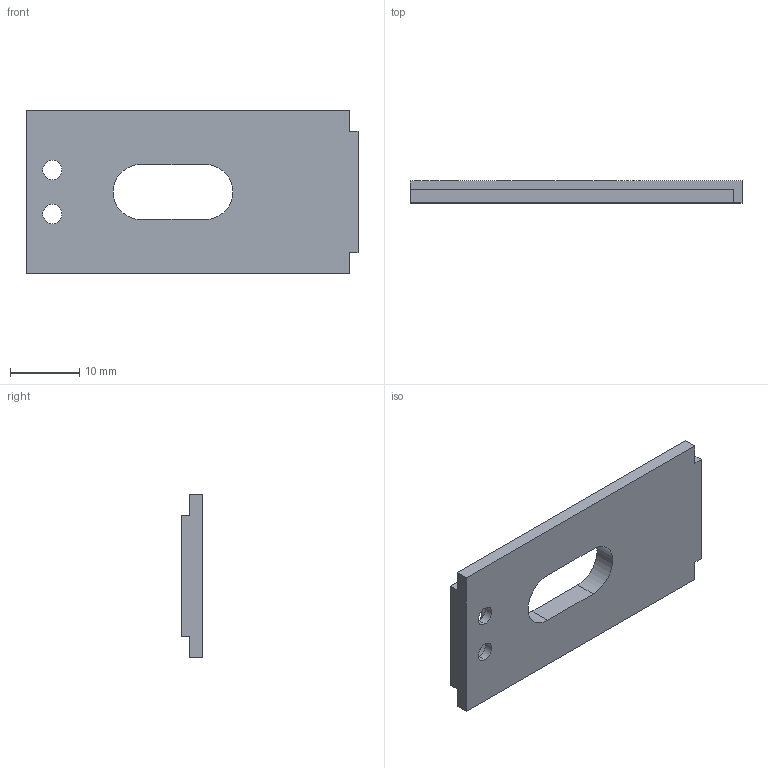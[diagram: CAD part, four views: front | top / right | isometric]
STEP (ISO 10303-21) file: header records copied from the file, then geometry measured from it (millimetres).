
FILE_DESCRIPTION (( 'STEP AP214' ), '1' );
FILE_NAME ('Original_Fire_Control_Well_Bottom.step', '2015-06-12T14:16:53', ( '' ), ( '' ), 'SwSTEP 2.0', 'SolidWorks 2015', '' );
FILE_SCHEMA (( 'AUTOMOTIVE_DESIGN' ));
Length unit declared in the file: inch
Products named in the file (1): Original_Fire_Control_Well_Bottom
Bounding box: 47.96 x 3.17 x 23.62 mm (x, y, z)
Volume: 2675.8 mm3; surface area: 2641.6 mm2
Topology: 1 solids, 1 shells, 26 faces, 69 edges, 46 vertices
Faces by surface type: plane 15, cylinder 11
Entity records: 867 total; most frequent: DIRECTION 145, CARTESIAN_POINT 142, ORIENTED_EDGE 138, EDGE_CURVE 69, AXIS2_PLACEMENT_3D 49, LINE 47, VECTOR 47, VERTEX_POINT 46
